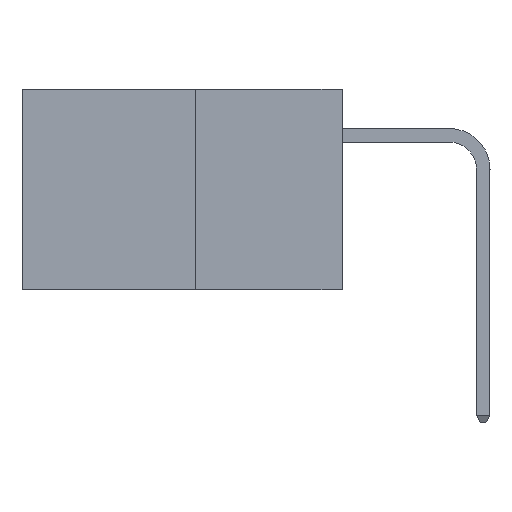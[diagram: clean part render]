
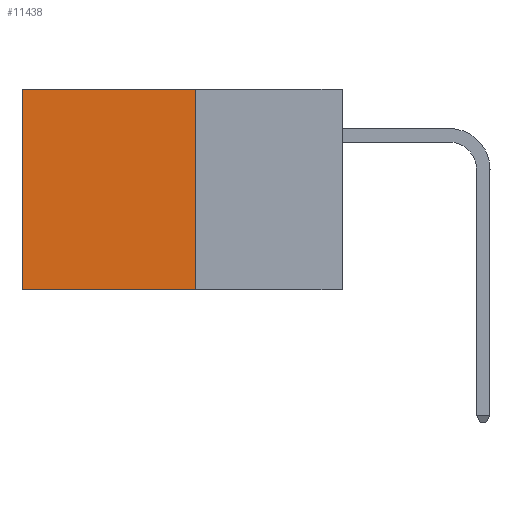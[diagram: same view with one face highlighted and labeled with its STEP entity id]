
A CAD part, left-side view. The second image highlights one B-rep face of the part: STEP entity #11438.
In plain terms, the highlighted planar face has unit normal (-1, 0, 0).
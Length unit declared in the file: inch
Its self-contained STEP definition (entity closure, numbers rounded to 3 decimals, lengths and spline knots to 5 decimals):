
#258 = EDGE_CURVE ( 'NONE', #6874, #15998, #7264, .T. ) ;
#765 = VECTOR ( 'NONE', #6488, 39.37008 ) ;
#1006 = CARTESIAN_POINT ( 'NONE',  ( 0.277, 0.59, -0.37 ) ) ;
#1380 = VECTOR ( 'NONE', #6825, 39.37008 ) ;
#1549 = VECTOR ( 'NONE', #6888, 39.37008 ) ;
#2121 = EDGE_CURVE ( 'NONE', #15998, #9893, #5976, .T. ) ;
#2359 = CARTESIAN_POINT ( 'NONE',  ( 0.277, 0.27, 0. ) ) ;
#2812 = ORIENTED_EDGE ( 'NONE', *, *, #6497, .F. ) ;
#3432 = PLANE ( 'NONE',  #15214 ) ;
#4052 = VERTEX_POINT ( 'NONE', #7419 ) ;
#4163 = CARTESIAN_POINT ( 'NONE',  ( 0.277, 0.27, -0.37 ) ) ;
#4721 = CARTESIAN_POINT ( 'NONE',  ( 0.277, 0.27, -0.37 ) ) ;
#4737 = CARTESIAN_POINT ( 'NONE',  ( 0.277, 0.59, -0.37 ) ) ;
#4741 = LINE ( 'NONE', #4163, #1380 ) ;
#4932 = LINE ( 'NONE', #5570, #1549 ) ;
#5377 = FACE_OUTER_BOUND ( 'NONE', #12374, .T. ) ;
#5570 = CARTESIAN_POINT ( 'NONE',  ( 0.277, 0.27, -0.37 ) ) ;
#5976 = LINE ( 'NONE', #4737, #11886 ) ;
#6076 = DIRECTION ( 'NONE',  ( 0., 0., -1. ) ) ;
#6488 = DIRECTION ( 'NONE',  ( 0., 1., 0. ) ) ;
#6497 = EDGE_CURVE ( 'NONE', #4052, #9893, #4741, .T. ) ;
#6825 = DIRECTION ( 'NONE',  ( 0., 1., 0. ) ) ;
#6874 = VERTEX_POINT ( 'NONE', #2359 ) ;
#6888 = DIRECTION ( 'NONE',  ( 0., 0., -1. ) ) ;
#7041 = DIRECTION ( 'NONE',  ( 0., 0., -1. ) ) ;
#7197 = ORIENTED_EDGE ( 'NONE', *, *, #258, .T. ) ;
#7264 = LINE ( 'NONE', #14934, #765 ) ;
#7419 = CARTESIAN_POINT ( 'NONE',  ( 0.277, 0.27, -0.37 ) ) ;
#7869 = ORIENTED_EDGE ( 'NONE', *, *, #12712, .F. ) ;
#8040 = CARTESIAN_POINT ( 'NONE',  ( 0.277, 0.59, 0. ) ) ;
#9500 = ORIENTED_EDGE ( 'NONE', *, *, #2121, .T. ) ;
#9893 = VERTEX_POINT ( 'NONE', #1006 ) ;
#11438 = ADVANCED_FACE ( 'NONE', ( #5377 ), #3432, .F. ) ;
#11886 = VECTOR ( 'NONE', #7041, 39.37008 ) ;
#12374 = EDGE_LOOP ( 'NONE', ( #9500, #2812, #7869, #7197 ) ) ;
#12712 = EDGE_CURVE ( 'NONE', #6874, #4052, #4932, .T. ) ;
#13526 = DIRECTION ( 'NONE',  ( 1., 0., 0. ) ) ;
#14934 = CARTESIAN_POINT ( 'NONE',  ( 0.277, 0.27, 0. ) ) ;
#15214 = AXIS2_PLACEMENT_3D ( 'NONE', #4721, #13526, #6076 ) ;
#15998 = VERTEX_POINT ( 'NONE', #8040 ) ;
